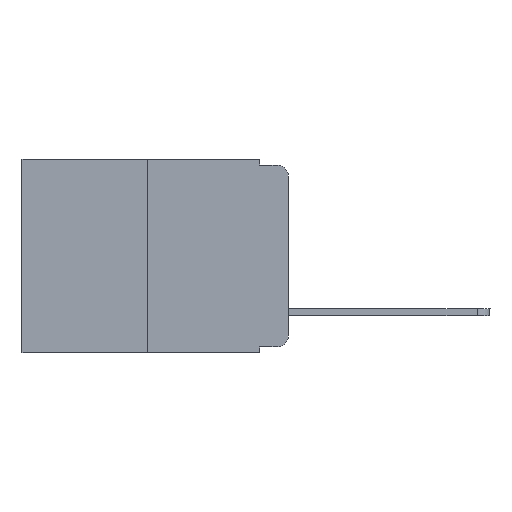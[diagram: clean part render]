
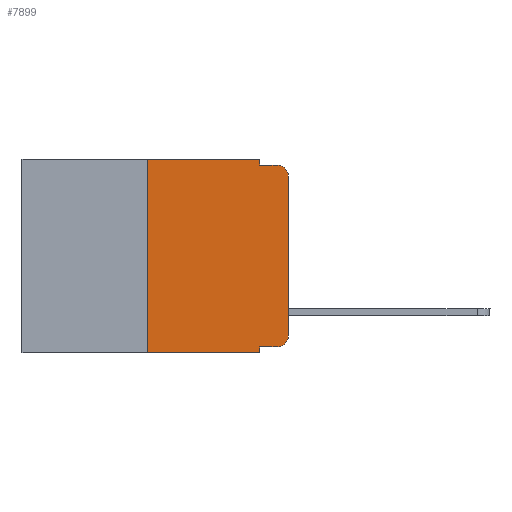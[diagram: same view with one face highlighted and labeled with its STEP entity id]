
A CAD part, left-side view. The second image highlights one B-rep face of the part: STEP entity #7899.
In plain terms, the highlighted planar face has unit normal (-1, 0, 0).
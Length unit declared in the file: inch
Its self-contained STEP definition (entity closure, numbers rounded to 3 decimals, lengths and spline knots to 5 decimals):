
#5 = AXIS2_PLACEMENT_3D ( 'NONE', #7614, #5323, #3812 ) ;
#189 = VECTOR ( 'NONE', #7844, 39.37008 ) ;
#504 = VERTEX_POINT ( 'NONE', #10289 ) ;
#516 = DIRECTION ( 'NONE',  ( 0., -1., 0. ) ) ;
#599 = CARTESIAN_POINT ( 'NONE',  ( 0., 0.02, -0.313 ) ) ;
#612 = ORIENTED_EDGE ( 'NONE', *, *, #2529, .T. ) ;
#661 = VERTEX_POINT ( 'NONE', #8239 ) ;
#867 = CARTESIAN_POINT ( 'NONE',  ( 0., 0., 0. ) ) ;
#1025 = EDGE_CURVE ( 'NONE', #8447, #1624, #9667, .T. ) ;
#1126 = ORIENTED_EDGE ( 'NONE', *, *, #2734, .T. ) ;
#1147 = DIRECTION ( 'NONE',  ( -1., 0., 0. ) ) ;
#1224 = DIRECTION ( 'NONE',  ( 0., -1., 0. ) ) ;
#1559 = LINE ( 'NONE', #6954, #189 ) ;
#1601 = DIRECTION ( 'NONE',  ( 0., 0., 1. ) ) ;
#1624 = VERTEX_POINT ( 'NONE', #9210 ) ;
#1795 = VECTOR ( 'NONE', #1224, 39.37008 ) ;
#1952 = LINE ( 'NONE', #4228, #1795 ) ;
#1967 = CARTESIAN_POINT ( 'NONE',  ( 0., 0.473, -0.343 ) ) ;
#2078 = LINE ( 'NONE', #1967, #7460 ) ;
#2117 = ORIENTED_EDGE ( 'NONE', *, *, #2454, .T. ) ;
#2220 = DIRECTION ( 'NONE',  ( 0., 0., -1. ) ) ;
#2223 = DIRECTION ( 'NONE',  ( 0., 0., -1. ) ) ;
#2345 = EDGE_CURVE ( 'NONE', #504, #8529, #10298, .T. ) ;
#2439 = VECTOR ( 'NONE', #1601, 39.37008 ) ;
#2454 = EDGE_CURVE ( 'NONE', #8373, #8447, #8837, .T. ) ;
#2526 = EDGE_LOOP ( 'NONE', ( #2117, #7616, #5453, #5037, #8667, #3605, #2884, #5140, #612, #1126 ) ) ;
#2529 = EDGE_CURVE ( 'NONE', #3419, #8603, #1952, .T. ) ;
#2668 = EDGE_CURVE ( 'NONE', #8529, #7198, #2937, .T. ) ;
#2734 = EDGE_CURVE ( 'NONE', #8603, #8373, #9089, .T. ) ;
#2884 = ORIENTED_EDGE ( 'NONE', *, *, #5294, .T. ) ;
#2937 = LINE ( 'NONE', #6894, #7419 ) ;
#2944 = LINE ( 'NONE', #7833, #3487 ) ;
#3419 = VERTEX_POINT ( 'NONE', #3425 ) ;
#3425 = CARTESIAN_POINT ( 'NONE',  ( 0., 0.051, -0.333 ) ) ;
#3487 = VECTOR ( 'NONE', #2220, 39.37008 ) ;
#3605 = ORIENTED_EDGE ( 'NONE', *, *, #2345, .F. ) ;
#3812 = DIRECTION ( 'NONE',  ( 0., 0., -1. ) ) ;
#3852 = CARTESIAN_POINT ( 'NONE',  ( 0., 0., -0.313 ) ) ;
#4055 = CARTESIAN_POINT ( 'NONE',  ( 0., 0., -0.03 ) ) ;
#4228 = CARTESIAN_POINT ( 'NONE',  ( 0., 0.051, -0.333 ) ) ;
#4502 = DIRECTION ( 'NONE',  ( -1., 0., 0. ) ) ;
#5037 = ORIENTED_EDGE ( 'NONE', *, *, #9284, .F. ) ;
#5140 = ORIENTED_EDGE ( 'NONE', *, *, #6366, .F. ) ;
#5294 = EDGE_CURVE ( 'NONE', #504, #661, #2078, .T. ) ;
#5323 = DIRECTION ( 'NONE',  ( 1., 0., 0. ) ) ;
#5453 = ORIENTED_EDGE ( 'NONE', *, *, #5904, .F. ) ;
#5820 = CARTESIAN_POINT ( 'NONE',  ( 0., 0.02, -0.03 ) ) ;
#5904 = EDGE_CURVE ( 'NONE', #9100, #1624, #1559, .T. ) ;
#6084 = AXIS2_PLACEMENT_3D ( 'NONE', #599, #4502, #7675 ) ;
#6170 = LINE ( 'NONE', #9365, #10010 ) ;
#6207 = DIRECTION ( 'NONE',  ( 0., -1., 0. ) ) ;
#6366 = EDGE_CURVE ( 'NONE', #3419, #661, #2944, .T. ) ;
#6852 = CARTESIAN_POINT ( 'NONE',  ( 0., 0.051, -0.01 ) ) ;
#6894 = CARTESIAN_POINT ( 'NONE',  ( 0., 0.473, 0. ) ) ;
#6954 = CARTESIAN_POINT ( 'NONE',  ( 0., 0.051, -0.01 ) ) ;
#7198 = VERTEX_POINT ( 'NONE', #10076 ) ;
#7419 = VECTOR ( 'NONE', #6207, 39.37008 ) ;
#7460 = VECTOR ( 'NONE', #516, 39.37008 ) ;
#7483 = CARTESIAN_POINT ( 'NONE',  ( 0., 0.02, -0.333 ) ) ;
#7614 = CARTESIAN_POINT ( 'NONE',  ( 0., 0.473, 0. ) ) ;
#7616 = ORIENTED_EDGE ( 'NONE', *, *, #1025, .T. ) ;
#7675 = DIRECTION ( 'NONE',  ( 0., 0., -1. ) ) ;
#7833 = CARTESIAN_POINT ( 'NONE',  ( 0., 0.051, 0. ) ) ;
#7844 = DIRECTION ( 'NONE',  ( 0., -1., 0. ) ) ;
#7899 = ADVANCED_FACE ( 'NONE', ( #10089 ), #9450, .F. ) ;
#8224 = CARTESIAN_POINT ( 'NONE',  ( 0., 0.25, 0. ) ) ;
#8239 = CARTESIAN_POINT ( 'NONE',  ( 0., 0.051, -0.343 ) ) ;
#8373 = VERTEX_POINT ( 'NONE', #3852 ) ;
#8447 = VERTEX_POINT ( 'NONE', #4055 ) ;
#8529 = VERTEX_POINT ( 'NONE', #8224 ) ;
#8603 = VERTEX_POINT ( 'NONE', #7483 ) ;
#8667 = ORIENTED_EDGE ( 'NONE', *, *, #2668, .F. ) ;
#8686 = CARTESIAN_POINT ( 'NONE',  ( 0., 0.25, 0. ) ) ;
#8733 = DIRECTION ( 'NONE',  ( 0., 0., 1. ) ) ;
#8837 = LINE ( 'NONE', #867, #2439 ) ;
#9089 = CIRCLE ( 'NONE', #6084, 0.02 ) ;
#9100 = VERTEX_POINT ( 'NONE', #6852 ) ;
#9210 = CARTESIAN_POINT ( 'NONE',  ( 0., 0.02, -0.01 ) ) ;
#9284 = EDGE_CURVE ( 'NONE', #7198, #9100, #6170, .T. ) ;
#9365 = CARTESIAN_POINT ( 'NONE',  ( 0., 0.051, 0. ) ) ;
#9450 = PLANE ( 'NONE',  #5 ) ;
#9475 = AXIS2_PLACEMENT_3D ( 'NONE', #5820, #1147, #9861 ) ;
#9667 = CIRCLE ( 'NONE', #9475, 0.02 ) ;
#9861 = DIRECTION ( 'NONE',  ( 0., 0., -1. ) ) ;
#10010 = VECTOR ( 'NONE', #2223, 39.37008 ) ;
#10076 = CARTESIAN_POINT ( 'NONE',  ( 0., 0.051, 0. ) ) ;
#10089 = FACE_OUTER_BOUND ( 'NONE', #2526, .T. ) ;
#10102 = VECTOR ( 'NONE', #8733, 39.37008 ) ;
#10289 = CARTESIAN_POINT ( 'NONE',  ( 0., 0.25, -0.343 ) ) ;
#10298 = LINE ( 'NONE', #8686, #10102 ) ;
